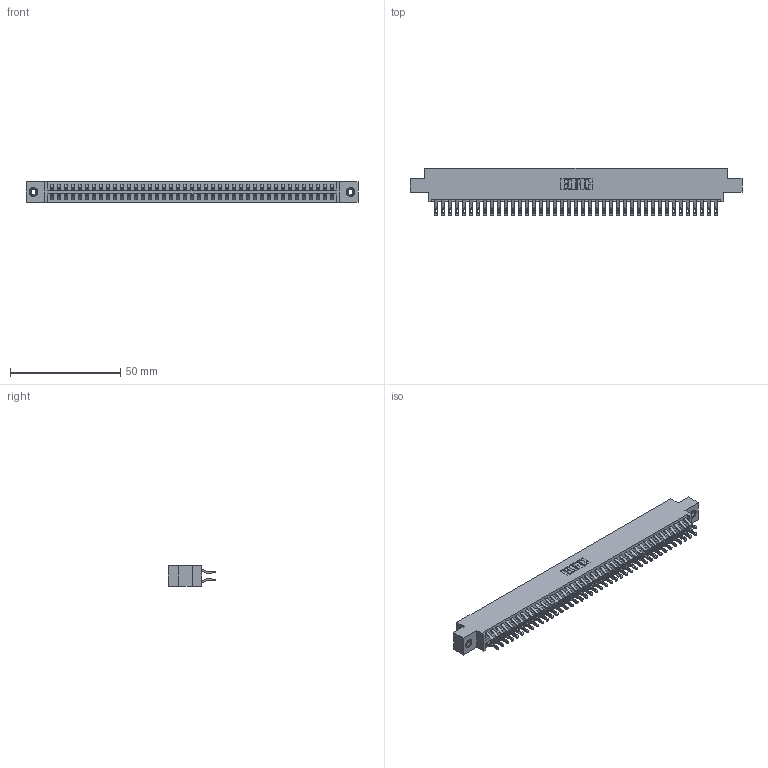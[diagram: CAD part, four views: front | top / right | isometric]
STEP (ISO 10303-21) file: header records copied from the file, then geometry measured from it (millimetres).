
FILE_DESCRIPTION (( 'STEP AP203' ), '1' );
FILE_NAME ('346-082-555-808.STEP', '2022-05-25T18:17:29', ( '' ), ( '' ), 'SwSTEP 2.0', 'SolidWorks 2020', '' );
FILE_SCHEMA (( 'CONFIG_CONTROL_DESIGN' ));
Length unit declared in the file: inch
Products named in the file (4): 345-292-001_555 Tail; 346-082-555-808; 346 Part_0.170 Offset - 0.156 Dia-TI; 345-250-001_345-250-003-102
Assembly tree (85 placements, depth 2):
  346-082-555-808
    346 Part_0.170 Offset - 0.156 Dia-TI
    345-292-001_555 Tail  x82
    345-250-001_345-250-003-102  x2
Bounding box: 150.75 x 21.46 x 9.4 mm (x, y, z)
Volume: 14768.8 mm3; surface area: 21332.5 mm2
Topology: 85 solids, 85 shells, 4942 faces, 15483 edges, 10314 vertices
Faces by surface type: plane 2818, cylinder 2108, cone 12, torus 4
Entity records: 28536 total; most frequent: CARTESIAN_POINT 4725, ORIENTED_EDGE 4622, DIRECTION 4209, EDGE_CURVE 2311, VECTOR 1975, LINE 1975, VERTEX_POINT 1536, AXIS2_PLACEMENT_3D 1117
